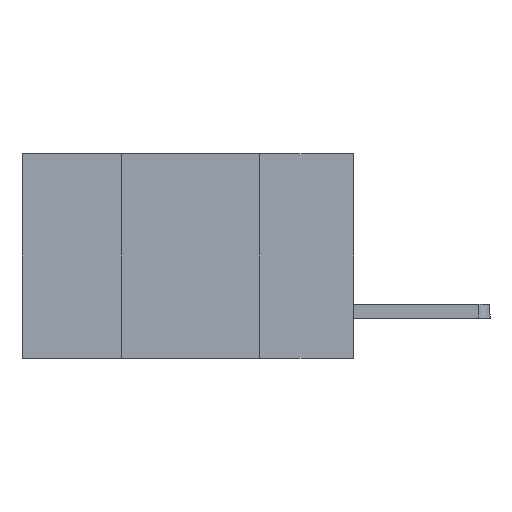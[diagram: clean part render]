
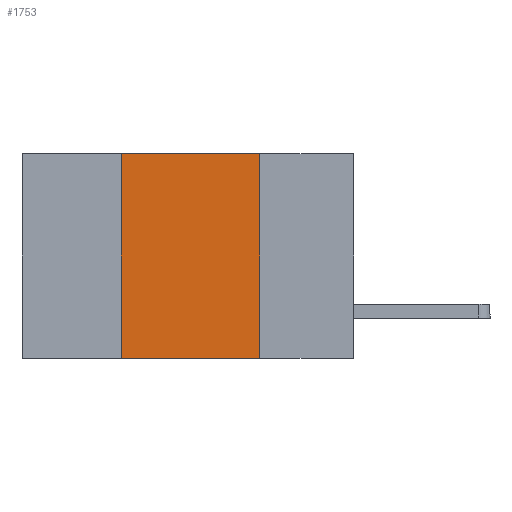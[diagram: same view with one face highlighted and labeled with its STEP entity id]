
A CAD part, left-side view. The second image highlights one B-rep face of the part: STEP entity #1753.
In plain terms, the highlighted planar face has unit normal (-1, 0, 0).
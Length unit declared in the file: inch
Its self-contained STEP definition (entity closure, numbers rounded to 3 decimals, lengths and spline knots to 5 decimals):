
#130 = DIRECTION ( 'NONE',  ( 0., 0., -1. ) ) ;
#435 = ORIENTED_EDGE ( 'NONE', *, *, #4897, .F. ) ;
#694 = ORIENTED_EDGE ( 'NONE', *, *, #1775, .F. ) ;
#1091 = VERTEX_POINT ( 'NONE', #8416 ) ;
#1672 = VERTEX_POINT ( 'NONE', #5042 ) ;
#1753 = ADVANCED_FACE ( 'NONE', ( #1973 ), #4830, .F. ) ;
#1775 = EDGE_CURVE ( 'NONE', #5857, #8761, #4974, .T. ) ;
#1973 = FACE_OUTER_BOUND ( 'NONE', #4797, .T. ) ;
#2087 = VECTOR ( 'NONE', #6792, 39.37008 ) ;
#3054 = LINE ( 'NONE', #5652, #8158 ) ;
#3278 = CARTESIAN_POINT ( 'NONE',  ( 0., 0.6, 0. ) ) ;
#3942 = VECTOR ( 'NONE', #130, 39.37008 ) ;
#4109 = LINE ( 'NONE', #3278, #2087 ) ;
#4754 = CARTESIAN_POINT ( 'NONE',  ( 0., 0.42, 0. ) ) ;
#4788 = ORIENTED_EDGE ( 'NONE', *, *, #7729, .T. ) ;
#4797 = EDGE_LOOP ( 'NONE', ( #6174, #435, #694, #4788 ) ) ;
#4830 = PLANE ( 'NONE',  #8910 ) ;
#4897 = EDGE_CURVE ( 'NONE', #8761, #1672, #4109, .T. ) ;
#4974 = LINE ( 'NONE', #4754, #7032 ) ;
#4983 = DIRECTION ( 'NONE',  ( 0., -1., 0. ) ) ;
#5042 = CARTESIAN_POINT ( 'NONE',  ( 0., 0.17, 0. ) ) ;
#5060 = CARTESIAN_POINT ( 'NONE',  ( 0., 0.6, 0. ) ) ;
#5078 = DIRECTION ( 'NONE',  ( 1., 0., 0. ) ) ;
#5421 = CARTESIAN_POINT ( 'NONE',  ( 0., 0.17, 0. ) ) ;
#5652 = CARTESIAN_POINT ( 'NONE',  ( 0., 0.6, -0.37 ) ) ;
#5857 = VERTEX_POINT ( 'NONE', #6181 ) ;
#5897 = CARTESIAN_POINT ( 'NONE',  ( 0., 0.42, 0. ) ) ;
#5922 = DIRECTION ( 'NONE',  ( 0., 0., 1. ) ) ;
#6174 = ORIENTED_EDGE ( 'NONE', *, *, #8941, .F. ) ;
#6181 = CARTESIAN_POINT ( 'NONE',  ( 0., 0.42, -0.37 ) ) ;
#6643 = DIRECTION ( 'NONE',  ( 0., 0., -1. ) ) ;
#6792 = DIRECTION ( 'NONE',  ( 0., -1., 0. ) ) ;
#7032 = VECTOR ( 'NONE', #5922, 39.37008 ) ;
#7729 = EDGE_CURVE ( 'NONE', #5857, #1091, #3054, .T. ) ;
#8158 = VECTOR ( 'NONE', #4983, 39.37008 ) ;
#8416 = CARTESIAN_POINT ( 'NONE',  ( 0., 0.17, -0.37 ) ) ;
#8761 = VERTEX_POINT ( 'NONE', #5897 ) ;
#8910 = AXIS2_PLACEMENT_3D ( 'NONE', #5060, #5078, #6643 ) ;
#8941 = EDGE_CURVE ( 'NONE', #1672, #1091, #9442, .T. ) ;
#9442 = LINE ( 'NONE', #5421, #3942 ) ;
